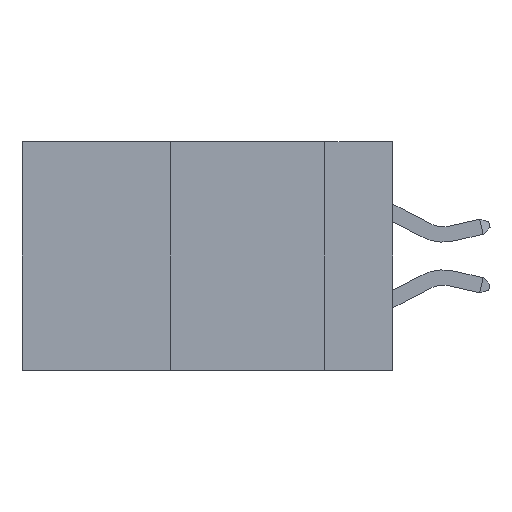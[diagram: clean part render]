
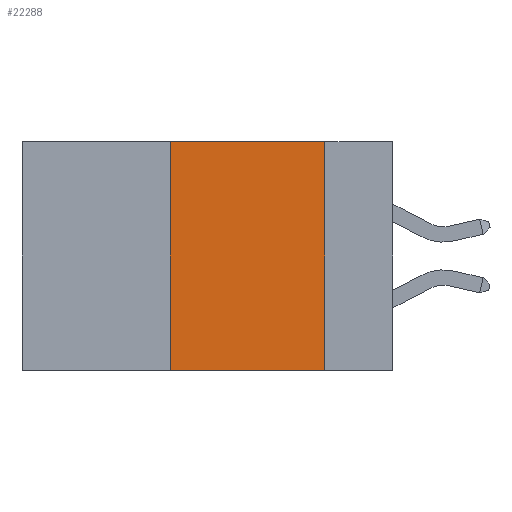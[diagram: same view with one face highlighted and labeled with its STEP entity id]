
A CAD part, left-side view. The second image highlights one B-rep face of the part: STEP entity #22288.
In plain terms, the highlighted planar face has unit normal (-1, 0, 0).
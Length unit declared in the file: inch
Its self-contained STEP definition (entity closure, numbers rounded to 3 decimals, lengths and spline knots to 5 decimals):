
#412 = FACE_OUTER_BOUND ( 'NONE', #20514, .T. ) ;
#1389 = DIRECTION ( 'NONE',  ( 0., -1., 0. ) ) ;
#2396 = VECTOR ( 'NONE', #1389, 39.37008 ) ;
#2991 = EDGE_CURVE ( 'NONE', #10655, #24624, #4216, .T. ) ;
#4120 = LINE ( 'NONE', #16234, #13653 ) ;
#4216 = LINE ( 'NONE', #22134, #16725 ) ;
#5407 = VERTEX_POINT ( 'NONE', #10077 ) ;
#6336 = CARTESIAN_POINT ( 'NONE',  ( 0., 0.11, -0.37 ) ) ;
#6474 = ORIENTED_EDGE ( 'NONE', *, *, #20013, .F. ) ;
#7985 = PLANE ( 'NONE',  #16263 ) ;
#10077 = CARTESIAN_POINT ( 'NONE',  ( 0., 0.36, 0. ) ) ;
#10249 = DIRECTION ( 'NONE',  ( 0., 0., -1. ) ) ;
#10485 = DIRECTION ( 'NONE',  ( 0., -1., 0. ) ) ;
#10655 = VERTEX_POINT ( 'NONE', #16842 ) ;
#12097 = EDGE_CURVE ( 'NONE', #19886, #24624, #12465, .T. ) ;
#12201 = DIRECTION ( 'NONE',  ( 0., 0., -1. ) ) ;
#12438 = CARTESIAN_POINT ( 'NONE',  ( 0., 0.36, -0.37 ) ) ;
#12465 = LINE ( 'NONE', #22232, #18199 ) ;
#13653 = VECTOR ( 'NONE', #18485, 39.37008 ) ;
#14064 = ORIENTED_EDGE ( 'NONE', *, *, #12097, .T. ) ;
#15920 = ORIENTED_EDGE ( 'NONE', *, *, #2991, .F. ) ;
#16234 = CARTESIAN_POINT ( 'NONE',  ( 0., 0.36, 0. ) ) ;
#16263 = AXIS2_PLACEMENT_3D ( 'NONE', #16293, #22098, #12201 ) ;
#16293 = CARTESIAN_POINT ( 'NONE',  ( 0., 0.6, 0. ) ) ;
#16725 = VECTOR ( 'NONE', #10249, 39.37008 ) ;
#16842 = CARTESIAN_POINT ( 'NONE',  ( 0., 0.11, 0. ) ) ;
#17177 = EDGE_CURVE ( 'NONE', #19886, #5407, #4120, .T. ) ;
#18199 = VECTOR ( 'NONE', #10485, 39.37008 ) ;
#18485 = DIRECTION ( 'NONE',  ( 0., 0., 1. ) ) ;
#19403 = CARTESIAN_POINT ( 'NONE',  ( 0., 0.6, 0. ) ) ;
#19886 = VERTEX_POINT ( 'NONE', #12438 ) ;
#20013 = EDGE_CURVE ( 'NONE', #5407, #10655, #22714, .T. ) ;
#20514 = EDGE_LOOP ( 'NONE', ( #15920, #6474, #25380, #14064 ) ) ;
#22098 = DIRECTION ( 'NONE',  ( 1., 0., 0. ) ) ;
#22134 = CARTESIAN_POINT ( 'NONE',  ( 0., 0.11, 0. ) ) ;
#22232 = CARTESIAN_POINT ( 'NONE',  ( 0., 0.6, -0.37 ) ) ;
#22288 = ADVANCED_FACE ( 'NONE', ( #412 ), #7985, .F. ) ;
#22714 = LINE ( 'NONE', #19403, #2396 ) ;
#24624 = VERTEX_POINT ( 'NONE', #6336 ) ;
#25380 = ORIENTED_EDGE ( 'NONE', *, *, #17177, .F. ) ;
